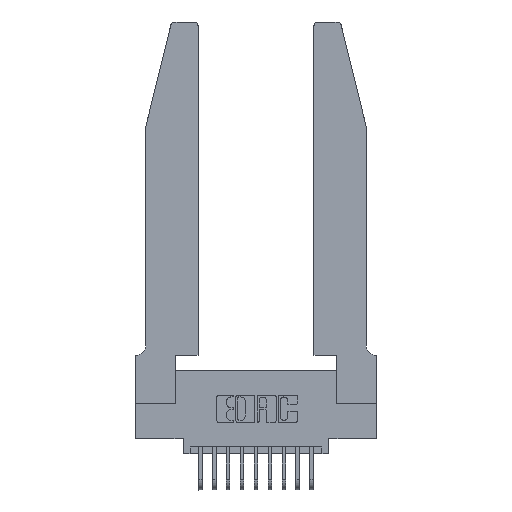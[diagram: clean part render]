
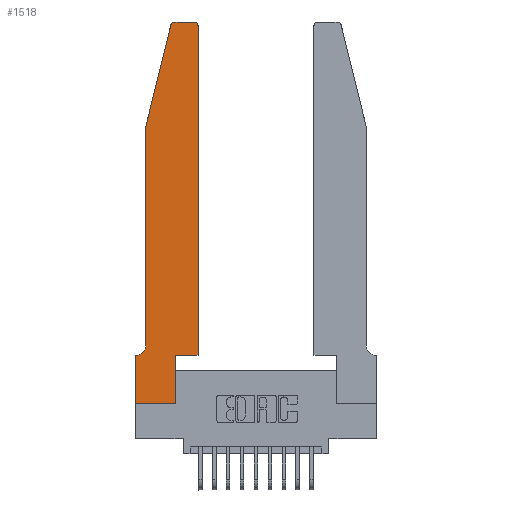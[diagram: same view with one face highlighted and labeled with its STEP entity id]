
A CAD part, top view. The second image highlights one B-rep face of the part: STEP entity #1518.
In plain terms, the highlighted planar face has unit normal (0, 0, 1).
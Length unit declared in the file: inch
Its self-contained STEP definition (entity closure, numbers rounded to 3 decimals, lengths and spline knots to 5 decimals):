
#216 = LINE ( 'NONE', #9098, #7029 ) ;
#415 = EDGE_CURVE ( 'NONE', #5897, #5017, #11394, .T. ) ;
#678 = DIRECTION ( 'NONE',  ( 0., -1., 0. ) ) ;
#1003 = CARTESIAN_POINT ( 'NONE',  ( 0.4505, 0.35, 0.37 ) ) ;
#1331 = CARTESIAN_POINT ( 'NONE',  ( 0.2605, 2.75, 0.37 ) ) ;
#1410 = CARTESIAN_POINT ( 'NONE',  ( 0.0755, 2., 0.37 ) ) ;
#1518 = ADVANCED_FACE ( 'NONE', ( #11928 ), #12358, .T. ) ;
#2025 = CARTESIAN_POINT ( 'NONE',  ( 0.4205, 2.72, 0.37 ) ) ;
#2041 = VECTOR ( 'NONE', #7388, 39.37008 ) ;
#2271 = CARTESIAN_POINT ( 'NONE',  ( 0., 0.35, 0.37 ) ) ;
#2453 = LINE ( 'NONE', #4733, #2041 ) ;
#2602 = DIRECTION ( 'NONE',  ( -1., 0., 0. ) ) ;
#2665 = EDGE_CURVE ( 'NONE', #6569, #11154, #2453, .T. ) ;
#2677 = ORIENTED_EDGE ( 'NONE', *, *, #8097, .T. ) ;
#2794 = EDGE_LOOP ( 'NONE', ( #7102, #6922, #14848, #2677, #10087, #8673, #13522, #10456, #10607, #13019, #12815, #12513 ) ) ;
#3013 = VERTEX_POINT ( 'NONE', #8333 ) ;
#3034 = CARTESIAN_POINT ( 'NONE',  ( 0.2865, 0.35, 0.37 ) ) ;
#3069 = VERTEX_POINT ( 'NONE', #12852 ) ;
#3070 = DIRECTION ( 'NONE',  ( -1., 0., 0. ) ) ;
#3184 = EDGE_CURVE ( 'NONE', #11154, #3069, #12451, .T. ) ;
#3187 = VECTOR ( 'NONE', #2602, 39.37008 ) ;
#3213 = CARTESIAN_POINT ( 'NONE',  ( 0., 0., 0.37 ) ) ;
#3303 = DIRECTION ( 'NONE',  ( 1., 0., 0. ) ) ;
#3538 = EDGE_CURVE ( 'NONE', #3013, #4499, #216, .T. ) ;
#3932 = CIRCLE ( 'NONE', #7525, 0.07 ) ;
#4208 = CARTESIAN_POINT ( 'NONE',  ( 0.4505, 0.35, 0.37 ) ) ;
#4460 = CARTESIAN_POINT ( 'NONE',  ( 0.0755, 2., 0.37 ) ) ;
#4499 = VERTEX_POINT ( 'NONE', #11219 ) ;
#4517 = DIRECTION ( 'NONE',  ( 0., 0., 1. ) ) ;
#4659 = CARTESIAN_POINT ( 'NONE',  ( 0.0755, 0.35, 0.37 ) ) ;
#4733 = CARTESIAN_POINT ( 'NONE',  ( 0.4505, 0.35, 0.37 ) ) ;
#5017 = VERTEX_POINT ( 'NONE', #2271 ) ;
#5427 = LINE ( 'NONE', #1410, #14912 ) ;
#5897 = VERTEX_POINT ( 'NONE', #12777 ) ;
#6033 = VERTEX_POINT ( 'NONE', #8105 ) ;
#6080 = DIRECTION ( 'NONE',  ( 1., 0., 0. ) ) ;
#6411 = DIRECTION ( 'NONE',  ( 0., 1., 0. ) ) ;
#6569 = VERTEX_POINT ( 'NONE', #14291 ) ;
#6727 = DIRECTION ( 'NONE',  ( 0., 0., -1. ) ) ;
#6922 = ORIENTED_EDGE ( 'NONE', *, *, #12516, .T. ) ;
#7015 = DIRECTION ( 'NONE',  ( -0.239, -0.971, 0. ) ) ;
#7029 = VECTOR ( 'NONE', #14738, 39.37008 ) ;
#7102 = ORIENTED_EDGE ( 'NONE', *, *, #12227, .T. ) ;
#7157 = VERTEX_POINT ( 'NONE', #13207 ) ;
#7162 = EDGE_CURVE ( 'NONE', #5017, #3013, #12829, .T. ) ;
#7388 = DIRECTION ( 'NONE',  ( 1., 0., 0. ) ) ;
#7525 = AXIS2_PLACEMENT_3D ( 'NONE', #14114, #6727, #15337 ) ;
#7770 = DIRECTION ( 'NONE',  ( 0., -1., 0. ) ) ;
#8097 = EDGE_CURVE ( 'NONE', #10495, #7157, #5427, .T. ) ;
#8105 = CARTESIAN_POINT ( 'NONE',  ( 0.25487, 2.72718, 0.37 ) ) ;
#8195 = DIRECTION ( 'NONE',  ( 0., 1., 0. ) ) ;
#8290 = VERTEX_POINT ( 'NONE', #11794 ) ;
#8333 = CARTESIAN_POINT ( 'NONE',  ( 0., 0., 0.37 ) ) ;
#8673 = ORIENTED_EDGE ( 'NONE', *, *, #415, .T. ) ;
#9098 = CARTESIAN_POINT ( 'NONE',  ( 0., 0., 0.37 ) ) ;
#9274 = VECTOR ( 'NONE', #7015, 39.37008 ) ;
#9434 = VECTOR ( 'NONE', #8195, 39.37008 ) ;
#9944 = LINE ( 'NONE', #1331, #3187 ) ;
#9963 = EDGE_CURVE ( 'NONE', #7157, #5897, #3932, .T. ) ;
#10087 = ORIENTED_EDGE ( 'NONE', *, *, #9963, .T. ) ;
#10456 = ORIENTED_EDGE ( 'NONE', *, *, #3538, .T. ) ;
#10495 = VERTEX_POINT ( 'NONE', #12698 ) ;
#10607 = ORIENTED_EDGE ( 'NONE', *, *, #10647, .T. ) ;
#10640 = VECTOR ( 'NONE', #3070, 39.37008 ) ;
#10647 = EDGE_CURVE ( 'NONE', #4499, #6569, #15912, .T. ) ;
#10760 = CIRCLE ( 'NONE', #14341, 0.03 ) ;
#10789 = EDGE_CURVE ( 'NONE', #3069, #11256, #10760, .T. ) ;
#10869 = DIRECTION ( 'NONE',  ( 0., 0., 1. ) ) ;
#11137 = AXIS2_PLACEMENT_3D ( 'NONE', #12503, #12286, #6080 ) ;
#11154 = VERTEX_POINT ( 'NONE', #4208 ) ;
#11219 = CARTESIAN_POINT ( 'NONE',  ( 0.2865, 0., 0.37 ) ) ;
#11256 = VERTEX_POINT ( 'NONE', #15552 ) ;
#11394 = LINE ( 'NONE', #4659, #10640 ) ;
#11794 = CARTESIAN_POINT ( 'NONE',  ( 0.284, 2.75, 0.37 ) ) ;
#11928 = FACE_OUTER_BOUND ( 'NONE', #2794, .T. ) ;
#11978 = CARTESIAN_POINT ( 'NONE',  ( 0.284, 2.72, 0.37 ) ) ;
#12218 = CIRCLE ( 'NONE', #15968, 0.03 ) ;
#12227 = EDGE_CURVE ( 'NONE', #11256, #8290, #9944, .T. ) ;
#12286 = DIRECTION ( 'NONE',  ( 0., 0., 1. ) ) ;
#12358 = PLANE ( 'NONE',  #11137 ) ;
#12451 = LINE ( 'NONE', #1003, #14566 ) ;
#12503 = CARTESIAN_POINT ( 'NONE',  ( 0., 0.35, 0.37 ) ) ;
#12513 = ORIENTED_EDGE ( 'NONE', *, *, #10789, .T. ) ;
#12516 = EDGE_CURVE ( 'NONE', #8290, #6033, #12218, .T. ) ;
#12698 = CARTESIAN_POINT ( 'NONE',  ( 0.0755, 2., 0.37 ) ) ;
#12777 = CARTESIAN_POINT ( 'NONE',  ( 0.0055, 0.35, 0.37 ) ) ;
#12815 = ORIENTED_EDGE ( 'NONE', *, *, #3184, .T. ) ;
#12829 = LINE ( 'NONE', #3213, #15680 ) ;
#12852 = CARTESIAN_POINT ( 'NONE',  ( 0.4505, 2.72, 0.37 ) ) ;
#13019 = ORIENTED_EDGE ( 'NONE', *, *, #2665, .T. ) ;
#13207 = CARTESIAN_POINT ( 'NONE',  ( 0.0755, 0.42, 0.37 ) ) ;
#13233 = DIRECTION ( 'NONE',  ( 1., 0., 0. ) ) ;
#13522 = ORIENTED_EDGE ( 'NONE', *, *, #7162, .T. ) ;
#14114 = CARTESIAN_POINT ( 'NONE',  ( 0.0055, 0.42, 0.37 ) ) ;
#14291 = CARTESIAN_POINT ( 'NONE',  ( 0.2865, 0.35, 0.37 ) ) ;
#14341 = AXIS2_PLACEMENT_3D ( 'NONE', #2025, #10869, #3303 ) ;
#14566 = VECTOR ( 'NONE', #6411, 39.37008 ) ;
#14738 = DIRECTION ( 'NONE',  ( 1., 0., 0. ) ) ;
#14848 = ORIENTED_EDGE ( 'NONE', *, *, #14866, .T. ) ;
#14866 = EDGE_CURVE ( 'NONE', #6033, #10495, #15755, .T. ) ;
#14912 = VECTOR ( 'NONE', #7770, 39.37008 ) ;
#15337 = DIRECTION ( 'NONE',  ( -1., 0., 0. ) ) ;
#15552 = CARTESIAN_POINT ( 'NONE',  ( 0.4205, 2.75, 0.37 ) ) ;
#15680 = VECTOR ( 'NONE', #678, 39.37008 ) ;
#15755 = LINE ( 'NONE', #4460, #9274 ) ;
#15912 = LINE ( 'NONE', #3034, #9434 ) ;
#15968 = AXIS2_PLACEMENT_3D ( 'NONE', #11978, #4517, #13233 ) ;
